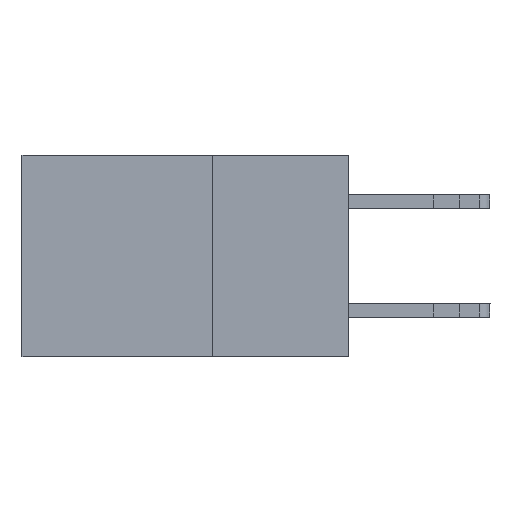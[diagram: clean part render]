
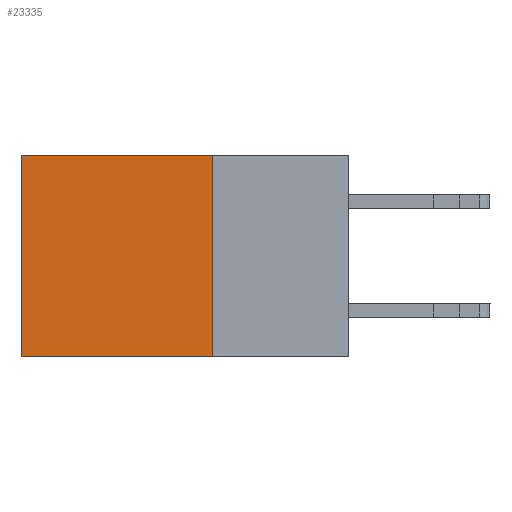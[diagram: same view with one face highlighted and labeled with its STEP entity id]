
A CAD part, left-side view. The second image highlights one B-rep face of the part: STEP entity #23335.
In plain terms, the highlighted planar face has unit normal (-1, 0, 0).
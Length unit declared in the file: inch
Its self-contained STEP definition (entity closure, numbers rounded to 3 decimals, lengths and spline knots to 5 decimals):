
#128 = EDGE_CURVE ( 'NONE', #5801, #7014, #7264, .T. ) ;
#1315 = CARTESIAN_POINT ( 'NONE',  ( 0.298, 0.6, -0.37 ) ) ;
#3416 = DIRECTION ( 'NONE',  ( 0., 0., -1. ) ) ;
#3569 = CARTESIAN_POINT ( 'NONE',  ( 0.298, 0.25, -0.37 ) ) ;
#5277 = EDGE_CURVE ( 'NONE', #11389, #19023, #25948, .T. ) ;
#5801 = VERTEX_POINT ( 'NONE', #25575 ) ;
#7014 = VERTEX_POINT ( 'NONE', #22945 ) ;
#7032 = EDGE_LOOP ( 'NONE', ( #14587, #13302, #17970, #8131 ) ) ;
#7264 = LINE ( 'NONE', #18800, #8550 ) ;
#8131 = ORIENTED_EDGE ( 'NONE', *, *, #128, .T. ) ;
#8381 = CARTESIAN_POINT ( 'NONE',  ( 0.298, 0.25, 0. ) ) ;
#8550 = VECTOR ( 'NONE', #22891, 39.37008 ) ;
#9142 = FACE_OUTER_BOUND ( 'NONE', #7032, .T. ) ;
#9205 = LINE ( 'NONE', #8381, #18835 ) ;
#10344 = DIRECTION ( 'NONE',  ( 0., 0., -1. ) ) ;
#10790 = PLANE ( 'NONE',  #19620 ) ;
#11059 = CARTESIAN_POINT ( 'NONE',  ( 0.298, 0.25, 0. ) ) ;
#11389 = VERTEX_POINT ( 'NONE', #21778 ) ;
#12048 = VECTOR ( 'NONE', #22250, 39.37008 ) ;
#13302 = ORIENTED_EDGE ( 'NONE', *, *, #5277, .F. ) ;
#14587 = ORIENTED_EDGE ( 'NONE', *, *, #17672, .T. ) ;
#17387 = EDGE_CURVE ( 'NONE', #5801, #11389, #9205, .T. ) ;
#17672 = EDGE_CURVE ( 'NONE', #7014, #19023, #23398, .T. ) ;
#17970 = ORIENTED_EDGE ( 'NONE', *, *, #17387, .F. ) ;
#18800 = CARTESIAN_POINT ( 'NONE',  ( 0.298, 0.25, 0. ) ) ;
#18835 = VECTOR ( 'NONE', #10344, 39.37008 ) ;
#19023 = VERTEX_POINT ( 'NONE', #1315 ) ;
#19277 = DIRECTION ( 'NONE',  ( 1., 0., 0. ) ) ;
#19620 = AXIS2_PLACEMENT_3D ( 'NONE', #11059, #19277, #21182 ) ;
#20071 = CARTESIAN_POINT ( 'NONE',  ( 0.298, 0.6, 0. ) ) ;
#20128 = VECTOR ( 'NONE', #3416, 39.37008 ) ;
#21182 = DIRECTION ( 'NONE',  ( 0., 0., -1. ) ) ;
#21778 = CARTESIAN_POINT ( 'NONE',  ( 0.298, 0.25, -0.37 ) ) ;
#22250 = DIRECTION ( 'NONE',  ( 0., 1., 0. ) ) ;
#22891 = DIRECTION ( 'NONE',  ( 0., 1., 0. ) ) ;
#22945 = CARTESIAN_POINT ( 'NONE',  ( 0.298, 0.6, 0. ) ) ;
#23335 = ADVANCED_FACE ( 'NONE', ( #9142 ), #10790, .F. ) ;
#23398 = LINE ( 'NONE', #20071, #20128 ) ;
#25575 = CARTESIAN_POINT ( 'NONE',  ( 0.298, 0.25, 0. ) ) ;
#25948 = LINE ( 'NONE', #3569, #12048 ) ;
